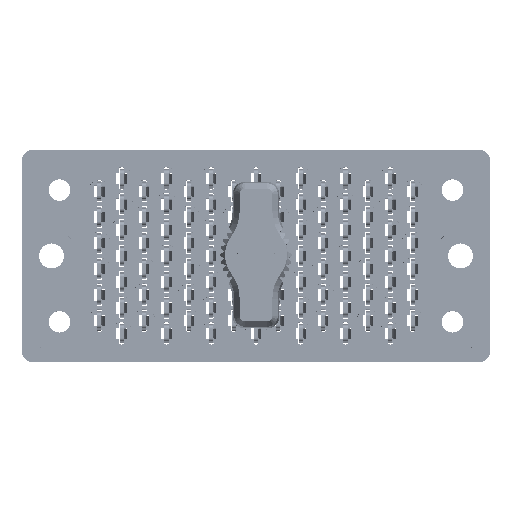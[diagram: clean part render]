
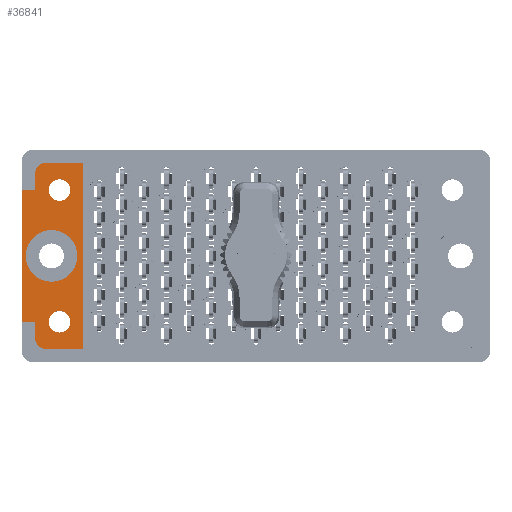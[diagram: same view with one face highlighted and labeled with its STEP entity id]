
A CAD part, top view. The second image highlights one B-rep face of the part: STEP entity #36841.
In plain terms, the highlighted planar face has unit normal (0, 0, 1).
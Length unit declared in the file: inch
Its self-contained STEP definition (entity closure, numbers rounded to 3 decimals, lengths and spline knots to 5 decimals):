
#1075 = EDGE_LOOP ( 'NONE', ( #4281, #65295 ) ) ;
#1314 = VERTEX_POINT ( 'NONE', #19972 ) ;
#1839 = PLANE ( 'NONE',  #20746 ) ;
#2271 = FACE_BOUND ( 'NONE', #54684, .T. ) ;
#3580 = FACE_BOUND ( 'NONE', #47274, .T. ) ;
#4034 = VECTOR ( 'NONE', #76044, 39.37008 ) ;
#4255 = VECTOR ( 'NONE', #83794, 39.37008 ) ;
#4281 = ORIENTED_EDGE ( 'NONE', *, *, #42260, .F. ) ;
#4799 = CARTESIAN_POINT ( 'NONE',  ( -1.2825, -0.478, -0.117 ) ) ;
#4865 = CARTESIAN_POINT ( 'NONE',  ( -1.359, 0.3825, -0.117 ) ) ;
#4993 = ORIENTED_EDGE ( 'NONE', *, *, #84980, .F. ) ;
#5135 = EDGE_CURVE ( 'NONE', #59018, #31457, #10528, .T. ) ;
#6813 = EDGE_CURVE ( 'NONE', #22183, #19094, #18977, .T. ) ;
#8752 = EDGE_CURVE ( 'NONE', #83812, #77241, #9170, .T. ) ;
#8850 = VERTEX_POINT ( 'NONE', #4799 ) ;
#9170 = CIRCLE ( 'NONE', #80980, 0.15 ) ;
#10528 = LINE ( 'NONE', #84154, #52577 ) ;
#10529 = EDGE_CURVE ( 'NONE', #23808, #21722, #31647, .T. ) ;
#11052 = AXIS2_PLACEMENT_3D ( 'NONE', #58589, #77994, #17593 ) ;
#11233 = DIRECTION ( 'NONE',  ( 0., 0., 1. ) ) ;
#13668 = CARTESIAN_POINT ( 'NONE',  ( -1.2035, 0.3825, -0.117 ) ) ;
#15486 = ORIENTED_EDGE ( 'NONE', *, *, #76609, .T. ) ;
#16018 = ORIENTED_EDGE ( 'NONE', *, *, #84489, .T. ) ;
#16857 = ORIENTED_EDGE ( 'NONE', *, *, #10529, .T. ) ;
#17034 = ORIENTED_EDGE ( 'NONE', *, *, #69238, .F. ) ;
#17593 = DIRECTION ( 'NONE',  ( 1., 0., 0. ) ) ;
#18722 = ORIENTED_EDGE ( 'NONE', *, *, #8752, .F. ) ;
#18742 = CIRCLE ( 'NONE', #58175, 0.0625 ) ;
#18977 = CIRCLE ( 'NONE', #51417, 0.062 ) ;
#19094 = VERTEX_POINT ( 'NONE', #35993 ) ;
#19285 = CIRCLE ( 'NONE', #20694, 0.15 ) ;
#19972 = CARTESIAN_POINT ( 'NONE',  ( -1.0785, 0.3825, -0.117 ) ) ;
#20141 = CIRCLE ( 'NONE', #44133, 0.062 ) ;
#20424 = CARTESIAN_POINT ( 'NONE',  ( -1.005, 0.54, -0.117 ) ) ;
#20613 = LINE ( 'NONE', #47491, #27369 ) ;
#20646 = VERTEX_POINT ( 'NONE', #36262 ) ;
#20694 = AXIS2_PLACEMENT_3D ( 'NONE', #63787, #84946, #37356 ) ;
#20746 = AXIS2_PLACEMENT_3D ( 'NONE', #82530, #22121, #49020 ) ;
#21685 = CARTESIAN_POINT ( 'NONE',  ( -1.359, -0.3825, -0.117 ) ) ;
#21722 = VERTEX_POINT ( 'NONE', #20424 ) ;
#22121 = DIRECTION ( 'NONE',  ( 0., 0., 1. ) ) ;
#22183 = VERTEX_POINT ( 'NONE', #47970 ) ;
#22451 = AXIS2_PLACEMENT_3D ( 'NONE', #85308, #11233, #72484 ) ;
#23808 = VERTEX_POINT ( 'NONE', #86606 ) ;
#27028 = DIRECTION ( 'NONE',  ( 0., -1., 0. ) ) ;
#27369 = VECTOR ( 'NONE', #48365, 39.37008 ) ;
#27419 = VERTEX_POINT ( 'NONE', #13668 ) ;
#27510 = ORIENTED_EDGE ( 'NONE', *, *, #38482, .F. ) ;
#28798 = ORIENTED_EDGE ( 'NONE', *, *, #45313, .T. ) ;
#30785 = VECTOR ( 'NONE', #27028, 39.37008 ) ;
#31457 = VERTEX_POINT ( 'NONE', #21685 ) ;
#31647 = LINE ( 'NONE', #57226, #66737 ) ;
#32024 = CIRCLE ( 'NONE', #81287, 0.0625 ) ;
#32238 = ORIENTED_EDGE ( 'NONE', *, *, #40380, .F. ) ;
#33797 = CARTESIAN_POINT ( 'NONE',  ( -1.2825, -0.3825, -0.117 ) ) ;
#33834 = DIRECTION ( 'NONE',  ( -1., 0., 0. ) ) ;
#35240 = ORIENTED_EDGE ( 'NONE', *, *, #6813, .T. ) ;
#35993 = CARTESIAN_POINT ( 'NONE',  ( -1.2825, 0.478, -0.117 ) ) ;
#36262 = CARTESIAN_POINT ( 'NONE',  ( -1.2035, -0.3825, -0.117 ) ) ;
#36384 = LINE ( 'NONE', #76926, #4034 ) ;
#36616 = CARTESIAN_POINT ( 'NONE',  ( 0., 0.3825, -0.117 ) ) ;
#36841 = ADVANCED_FACE ( 'NONE', ( #63980, #3580, #2271, #42400 ), #1839, .T. ) ;
#37356 = DIRECTION ( 'NONE',  ( 1., 0., 0. ) ) ;
#37770 = EDGE_CURVE ( 'NONE', #72937, #8850, #81228, .T. ) ;
#37944 = VERTEX_POINT ( 'NONE', #84717 ) ;
#38482 = EDGE_CURVE ( 'NONE', #1314, #27419, #42081, .T. ) ;
#38774 = VERTEX_POINT ( 'NONE', #81338 ) ;
#40173 = ORIENTED_EDGE ( 'NONE', *, *, #58199, .T. ) ;
#40380 = EDGE_CURVE ( 'NONE', #77241, #83812, #19285, .T. ) ;
#41762 = CARTESIAN_POINT ( 'NONE',  ( -1.2205, 0.478, -0.117 ) ) ;
#42081 = CIRCLE ( 'NONE', #11052, 0.0625 ) ;
#42260 = EDGE_CURVE ( 'NONE', #20646, #59346, #32024, .T. ) ;
#42400 = FACE_OUTER_BOUND ( 'NONE', #48842, .T. ) ;
#43497 = DIRECTION ( 'NONE',  ( 0., 0., 1. ) ) ;
#43932 = CARTESIAN_POINT ( 'NONE',  ( -1.141, -0.3825, -0.117 ) ) ;
#44133 = AXIS2_PLACEMENT_3D ( 'NONE', #82115, #81227, #48154 ) ;
#45313 = EDGE_CURVE ( 'NONE', #19094, #38774, #79396, .T. ) ;
#47274 = EDGE_LOOP ( 'NONE', ( #4993, #27510 ) ) ;
#47483 = CARTESIAN_POINT ( 'NONE',  ( 0., -0.3825, -0.117 ) ) ;
#47491 = CARTESIAN_POINT ( 'NONE',  ( 0., -0.54, -0.117 ) ) ;
#47714 = CARTESIAN_POINT ( 'NONE',  ( -1.2825, 0., -0.117 ) ) ;
#47970 = CARTESIAN_POINT ( 'NONE',  ( -1.2205, 0.54, -0.117 ) ) ;
#48154 = DIRECTION ( 'NONE',  ( 1., 0., 0. ) ) ;
#48199 = EDGE_CURVE ( 'NONE', #72937, #31457, #48357, .T. ) ;
#48357 = LINE ( 'NONE', #47483, #53704 ) ;
#48365 = DIRECTION ( 'NONE',  ( -1., 0., 0. ) ) ;
#48842 = EDGE_LOOP ( 'NONE', ( #55974, #40173, #17034, #16857, #15486, #35240, #28798, #16018, #57420, #75957 ) ) ;
#49020 = DIRECTION ( 'NONE',  ( 1., 0., 0. ) ) ;
#50037 = DIRECTION ( 'NONE',  ( 0., 0., 1. ) ) ;
#51417 = AXIS2_PLACEMENT_3D ( 'NONE', #41762, #76566, #67754 ) ;
#51471 = DIRECTION ( 'NONE',  ( 0., 1., 0. ) ) ;
#52577 = VECTOR ( 'NONE', #63422, 39.37008 ) ;
#53704 = VECTOR ( 'NONE', #33834, 39.37008 ) ;
#54684 = EDGE_LOOP ( 'NONE', ( #32238, #18722 ) ) ;
#55579 = CARTESIAN_POINT ( 'NONE',  ( -1.1875, 0., -0.117 ) ) ;
#55974 = ORIENTED_EDGE ( 'NONE', *, *, #37770, .T. ) ;
#57226 = CARTESIAN_POINT ( 'NONE',  ( -1.005, 0.617, -0.117 ) ) ;
#57420 = ORIENTED_EDGE ( 'NONE', *, *, #5135, .T. ) ;
#58175 = AXIS2_PLACEMENT_3D ( 'NONE', #43932, #43497, #70363 ) ;
#58199 = EDGE_CURVE ( 'NONE', #8850, #37944, #20141, .T. ) ;
#58519 = EDGE_CURVE ( 'NONE', #59346, #20646, #18742, .T. ) ;
#58589 = CARTESIAN_POINT ( 'NONE',  ( -1.141, 0.3825, -0.117 ) ) ;
#59018 = VERTEX_POINT ( 'NONE', #4865 ) ;
#59346 = VERTEX_POINT ( 'NONE', #77112 ) ;
#63422 = DIRECTION ( 'NONE',  ( 0., -1., 0. ) ) ;
#63787 = CARTESIAN_POINT ( 'NONE',  ( -1.1875, 0., -0.117 ) ) ;
#63811 = CARTESIAN_POINT ( 'NONE',  ( -1.3375, 0., -0.117 ) ) ;
#63980 = FACE_BOUND ( 'NONE', #1075, .T. ) ;
#64772 = DIRECTION ( 'NONE',  ( 1., 0., 0. ) ) ;
#64871 = DIRECTION ( 'NONE',  ( 0., -1., 0. ) ) ;
#65295 = ORIENTED_EDGE ( 'NONE', *, *, #58519, .F. ) ;
#66737 = VECTOR ( 'NONE', #51471, 39.37008 ) ;
#67754 = DIRECTION ( 'NONE',  ( 1., 0., 0. ) ) ;
#69203 = DIRECTION ( 'NONE',  ( 0., 0., 1. ) ) ;
#69238 = EDGE_CURVE ( 'NONE', #23808, #37944, #20613, .T. ) ;
#70102 = LINE ( 'NONE', #36616, #4255 ) ;
#70363 = DIRECTION ( 'NONE',  ( 1., 0., 0. ) ) ;
#70738 = DIRECTION ( 'NONE',  ( 1., 0., 0. ) ) ;
#72484 = DIRECTION ( 'NONE',  ( 1., 0., 0. ) ) ;
#72937 = VERTEX_POINT ( 'NONE', #33797 ) ;
#75957 = ORIENTED_EDGE ( 'NONE', *, *, #48199, .F. ) ;
#76044 = DIRECTION ( 'NONE',  ( -1., 0., 0. ) ) ;
#76566 = DIRECTION ( 'NONE',  ( 0., 0., 1. ) ) ;
#76609 = EDGE_CURVE ( 'NONE', #21722, #22183, #36384, .T. ) ;
#76926 = CARTESIAN_POINT ( 'NONE',  ( 0., 0.54, -0.117 ) ) ;
#77112 = CARTESIAN_POINT ( 'NONE',  ( -1.0785, -0.3825, -0.117 ) ) ;
#77241 = VERTEX_POINT ( 'NONE', #81058 ) ;
#77994 = DIRECTION ( 'NONE',  ( 0., 0., 1. ) ) ;
#78948 = CIRCLE ( 'NONE', #22451, 0.0625 ) ;
#78956 = CARTESIAN_POINT ( 'NONE',  ( -1.2825, 0., -0.117 ) ) ;
#79396 = LINE ( 'NONE', #78956, #81652 ) ;
#80980 = AXIS2_PLACEMENT_3D ( 'NONE', #55579, #69203, #64772 ) ;
#81058 = CARTESIAN_POINT ( 'NONE',  ( -1.0375, 0., -0.117 ) ) ;
#81227 = DIRECTION ( 'NONE',  ( 0., 0., 1. ) ) ;
#81228 = LINE ( 'NONE', #47714, #30785 ) ;
#81287 = AXIS2_PLACEMENT_3D ( 'NONE', #83543, #50037, #70738 ) ;
#81338 = CARTESIAN_POINT ( 'NONE',  ( -1.2825, 0.3825, -0.117 ) ) ;
#81652 = VECTOR ( 'NONE', #64871, 39.37008 ) ;
#82115 = CARTESIAN_POINT ( 'NONE',  ( -1.2205, -0.478, -0.117 ) ) ;
#82530 = CARTESIAN_POINT ( 'NONE',  ( -1.359, -0.617, -0.117 ) ) ;
#83543 = CARTESIAN_POINT ( 'NONE',  ( -1.141, -0.3825, -0.117 ) ) ;
#83794 = DIRECTION ( 'NONE',  ( -1., 0., 0. ) ) ;
#83812 = VERTEX_POINT ( 'NONE', #63811 ) ;
#84154 = CARTESIAN_POINT ( 'NONE',  ( -1.359, 0.617, -0.117 ) ) ;
#84489 = EDGE_CURVE ( 'NONE', #38774, #59018, #70102, .T. ) ;
#84717 = CARTESIAN_POINT ( 'NONE',  ( -1.2205, -0.54, -0.117 ) ) ;
#84946 = DIRECTION ( 'NONE',  ( 0., 0., 1. ) ) ;
#84980 = EDGE_CURVE ( 'NONE', #27419, #1314, #78948, .T. ) ;
#85308 = CARTESIAN_POINT ( 'NONE',  ( -1.141, 0.3825, -0.117 ) ) ;
#86606 = CARTESIAN_POINT ( 'NONE',  ( -1.005, -0.54, -0.117 ) ) ;
